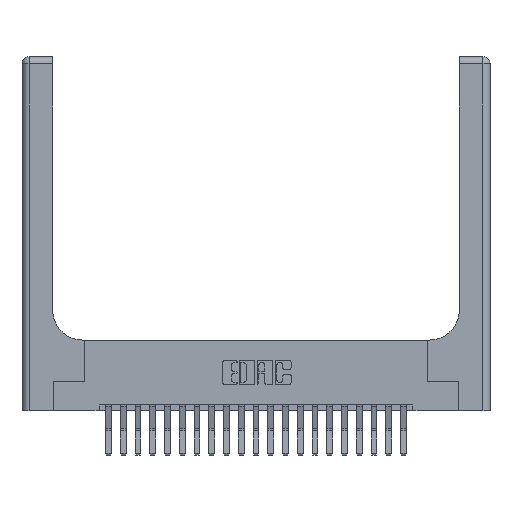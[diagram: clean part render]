
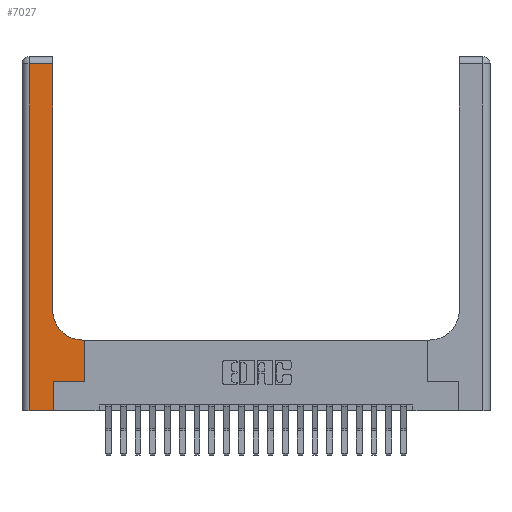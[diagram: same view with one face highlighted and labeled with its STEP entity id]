
A CAD part, top view. The second image highlights one B-rep face of the part: STEP entity #7027.
In plain terms, the highlighted planar face has unit normal (0, 0, 1).
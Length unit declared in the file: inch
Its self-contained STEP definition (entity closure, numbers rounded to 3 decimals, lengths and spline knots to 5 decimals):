
#144 = CARTESIAN_POINT ( 'NONE',  ( 0.265, 0., 0.37 ) ) ;
#145 = EDGE_CURVE ( 'NONE', #12178, #18442, #6259, .T. ) ;
#176 = CARTESIAN_POINT ( 'NONE',  ( 0., 3., 0.37 ) ) ;
#1538 = ORIENTED_EDGE ( 'NONE', *, *, #13864, .T. ) ;
#1738 = CARTESIAN_POINT ( 'NONE',  ( 0.06, 3., 0.37 ) ) ;
#1973 = LINE ( 'NONE', #9974, #7770 ) ;
#2300 = CARTESIAN_POINT ( 'NONE',  ( 0.265, 0., 0.37 ) ) ;
#2390 = FACE_OUTER_BOUND ( 'NONE', #20360, .T. ) ;
#2525 = VECTOR ( 'NONE', #14330, 39.37008 ) ;
#2533 = CIRCLE ( 'NONE', #6223, 0.25 ) ;
#3110 = CARTESIAN_POINT ( 'NONE',  ( 0.06, 0., 0.37 ) ) ;
#3898 = EDGE_CURVE ( 'NONE', #13065, #12925, #21557, .T. ) ;
#4729 = CARTESIAN_POINT ( 'NONE',  ( 0.51, 0.6, 0.37 ) ) ;
#5364 = LINE ( 'NONE', #7338, #10930 ) ;
#5408 = ORIENTED_EDGE ( 'NONE', *, *, #13312, .T. ) ;
#5635 = EDGE_CURVE ( 'NONE', #7203, #13065, #5364, .T. ) ;
#5794 = VERTEX_POINT ( 'NONE', #3110 ) ;
#6061 = CARTESIAN_POINT ( 'NONE',  ( 0.51, 0.85, 0.37 ) ) ;
#6102 = CARTESIAN_POINT ( 'NONE',  ( 0.06, 2.94, 0.37 ) ) ;
#6128 = DIRECTION ( 'NONE',  ( 1., 0., 0. ) ) ;
#6223 = AXIS2_PLACEMENT_3D ( 'NONE', #6061, #21033, #6128 ) ;
#6259 = LINE ( 'NONE', #20970, #2525 ) ;
#6734 = CARTESIAN_POINT ( 'NONE',  ( 0.265, 0.25, 0.37 ) ) ;
#7027 = ADVANCED_FACE ( 'NONE', ( #2390 ), #20295, .F. ) ;
#7203 = VERTEX_POINT ( 'NONE', #12552 ) ;
#7255 = VECTOR ( 'NONE', #8516, 39.37008 ) ;
#7338 = CARTESIAN_POINT ( 'NONE',  ( 0.26, 3., 0.37 ) ) ;
#7770 = VECTOR ( 'NONE', #18415, 39.37008 ) ;
#7855 = ORIENTED_EDGE ( 'NONE', *, *, #18557, .T. ) ;
#8458 = VERTEX_POINT ( 'NONE', #2300 ) ;
#8516 = DIRECTION ( 'NONE',  ( 0., -1., 0. ) ) ;
#9012 = DIRECTION ( 'NONE',  ( 0., 1., 0. ) ) ;
#9375 = ORIENTED_EDGE ( 'NONE', *, *, #13311, .T. ) ;
#9974 = CARTESIAN_POINT ( 'NONE',  ( 0.26, 0.6, 0.37 ) ) ;
#10142 = DIRECTION ( 'NONE',  ( 1., 0., 0. ) ) ;
#10565 = LINE ( 'NONE', #144, #15839 ) ;
#10731 = CARTESIAN_POINT ( 'NONE',  ( 0., 2.94, 0.37 ) ) ;
#10930 = VECTOR ( 'NONE', #9012, 39.37008 ) ;
#11209 = VECTOR ( 'NONE', #10142, 39.37008 ) ;
#11449 = ORIENTED_EDGE ( 'NONE', *, *, #20735, .T. ) ;
#11514 = AXIS2_PLACEMENT_3D ( 'NONE', #176, #20440, #18631 ) ;
#11712 = VECTOR ( 'NONE', #17161, 39.37008 ) ;
#11781 = CARTESIAN_POINT ( 'NONE',  ( 0., 0., 0.37 ) ) ;
#11983 = LINE ( 'NONE', #20524, #11712 ) ;
#12178 = VERTEX_POINT ( 'NONE', #17084 ) ;
#12404 = EDGE_CURVE ( 'NONE', #16579, #7203, #2533, .T. ) ;
#12552 = CARTESIAN_POINT ( 'NONE',  ( 0.26, 0.85, 0.37 ) ) ;
#12925 = VERTEX_POINT ( 'NONE', #6102 ) ;
#13065 = VERTEX_POINT ( 'NONE', #21704 ) ;
#13311 = EDGE_CURVE ( 'NONE', #5794, #8458, #16240, .T. ) ;
#13312 = EDGE_CURVE ( 'NONE', #12925, #5794, #19657, .T. ) ;
#13455 = ORIENTED_EDGE ( 'NONE', *, *, #12404, .T. ) ;
#13747 = ORIENTED_EDGE ( 'NONE', *, *, #145, .T. ) ;
#13864 = EDGE_CURVE ( 'NONE', #18442, #16579, #1973, .T. ) ;
#14330 = DIRECTION ( 'NONE',  ( 0., 1., 0. ) ) ;
#14866 = CARTESIAN_POINT ( 'NONE',  ( 0.528, 0.6, 0.37 ) ) ;
#15595 = DIRECTION ( 'NONE',  ( -1., 0., 0. ) ) ;
#15839 = VECTOR ( 'NONE', #18737, 39.37008 ) ;
#16240 = LINE ( 'NONE', #11781, #11209 ) ;
#16579 = VERTEX_POINT ( 'NONE', #4729 ) ;
#17084 = CARTESIAN_POINT ( 'NONE',  ( 0.528, 0.25, 0.37 ) ) ;
#17104 = VECTOR ( 'NONE', #15595, 39.37008 ) ;
#17161 = DIRECTION ( 'NONE',  ( 1., 0., 0. ) ) ;
#18415 = DIRECTION ( 'NONE',  ( -1., 0., 0. ) ) ;
#18442 = VERTEX_POINT ( 'NONE', #14866 ) ;
#18557 = EDGE_CURVE ( 'NONE', #19591, #12178, #11983, .T. ) ;
#18631 = DIRECTION ( 'NONE',  ( -1., 0., 0. ) ) ;
#18737 = DIRECTION ( 'NONE',  ( 0., 1., 0. ) ) ;
#18956 = ORIENTED_EDGE ( 'NONE', *, *, #3898, .T. ) ;
#19591 = VERTEX_POINT ( 'NONE', #6734 ) ;
#19657 = LINE ( 'NONE', #1738, #7255 ) ;
#20181 = ORIENTED_EDGE ( 'NONE', *, *, #5635, .T. ) ;
#20295 = PLANE ( 'NONE',  #11514 ) ;
#20360 = EDGE_LOOP ( 'NONE', ( #20181, #18956, #5408, #9375, #11449, #7855, #13747, #1538, #13455 ) ) ;
#20440 = DIRECTION ( 'NONE',  ( 0., 0., -1. ) ) ;
#20524 = CARTESIAN_POINT ( 'NONE',  ( 0.265, 0.25, 0.37 ) ) ;
#20735 = EDGE_CURVE ( 'NONE', #8458, #19591, #10565, .T. ) ;
#20970 = CARTESIAN_POINT ( 'NONE',  ( 0.528, 0.25, 0.37 ) ) ;
#21033 = DIRECTION ( 'NONE',  ( 0., 0., -1. ) ) ;
#21557 = LINE ( 'NONE', #10731, #17104 ) ;
#21704 = CARTESIAN_POINT ( 'NONE',  ( 0.26, 2.94, 0.37 ) ) ;
